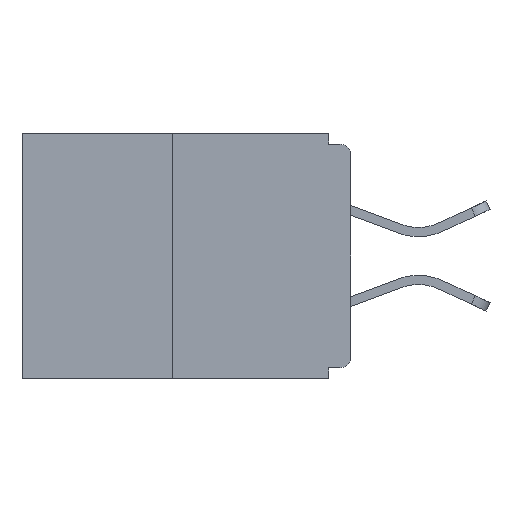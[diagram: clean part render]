
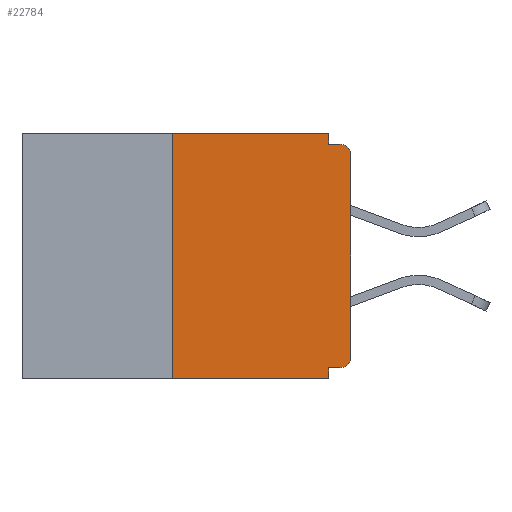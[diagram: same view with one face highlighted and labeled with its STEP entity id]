
A CAD part, left-side view. The second image highlights one B-rep face of the part: STEP entity #22784.
In plain terms, the highlighted planar face has unit normal (-1, 0, 0).
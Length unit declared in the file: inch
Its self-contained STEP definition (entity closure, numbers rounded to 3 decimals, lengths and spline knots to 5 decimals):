
#1736 = VECTOR ( 'NONE', #16011, 39.37008 ) ;
#2512 = EDGE_CURVE ( 'NONE', #23177, #23229, #24678, .T. ) ;
#2514 = CARTESIAN_POINT ( 'NONE',  ( 0., 0., -0.328 ) ) ;
#2651 = ORIENTED_EDGE ( 'NONE', *, *, #11335, .T. ) ;
#2685 = VERTEX_POINT ( 'NONE', #9331 ) ;
#2817 = VECTOR ( 'NONE', #18271, 39.37008 ) ;
#3033 = CARTESIAN_POINT ( 'NONE',  ( 0., 0.46, 0. ) ) ;
#3277 = CARTESIAN_POINT ( 'NONE',  ( 0., 0., -0.015 ) ) ;
#3321 = FACE_OUTER_BOUND ( 'NONE', #11960, .T. ) ;
#3941 = VECTOR ( 'NONE', #11304, 39.37008 ) ;
#3977 = ORIENTED_EDGE ( 'NONE', *, *, #21995, .T. ) ;
#4447 = CARTESIAN_POINT ( 'NONE',  ( 0., 0.25, 0. ) ) ;
#5215 = LINE ( 'NONE', #18017, #1736 ) ;
#5472 = DIRECTION ( 'NONE',  ( 0., 0., -1. ) ) ;
#5698 = CARTESIAN_POINT ( 'NONE',  ( 0., 0., -0.313 ) ) ;
#6737 = VECTOR ( 'NONE', #20362, 39.37008 ) ;
#7822 = CARTESIAN_POINT ( 'NONE',  ( 0., 0.031, -0.015 ) ) ;
#7859 = CIRCLE ( 'NONE', #24499, 0.015 ) ;
#7979 = DIRECTION ( 'NONE',  ( 0., 0., -1. ) ) ;
#8328 = LINE ( 'NONE', #17872, #12357 ) ;
#8707 = VERTEX_POINT ( 'NONE', #10016 ) ;
#8752 = VECTOR ( 'NONE', #18551, 39.37008 ) ;
#8835 = DIRECTION ( 'NONE',  ( 0., -1., 0. ) ) ;
#9174 = CARTESIAN_POINT ( 'NONE',  ( 0., 0., -0.03 ) ) ;
#9191 = EDGE_CURVE ( 'NONE', #17887, #13040, #24194, .T. ) ;
#9331 = CARTESIAN_POINT ( 'NONE',  ( 0., 0.031, 0. ) ) ;
#9357 = CARTESIAN_POINT ( 'NONE',  ( 0., 0.031, -0.343 ) ) ;
#9508 = VERTEX_POINT ( 'NONE', #5698 ) ;
#9536 = CARTESIAN_POINT ( 'NONE',  ( 0., 0.015, -0.03 ) ) ;
#10016 = CARTESIAN_POINT ( 'NONE',  ( 0., 0.015, -0.015 ) ) ;
#10813 = LINE ( 'NONE', #3277, #3941 ) ;
#11076 = DIRECTION ( 'NONE',  ( -1., 0., 0. ) ) ;
#11100 = PLANE ( 'NONE',  #22730 ) ;
#11304 = DIRECTION ( 'NONE',  ( 0., -1., 0. ) ) ;
#11315 = VECTOR ( 'NONE', #25258, 39.37008 ) ;
#11335 = EDGE_CURVE ( 'NONE', #22792, #8707, #7859, .T. ) ;
#11513 = CIRCLE ( 'NONE', #14159, 0.015 ) ;
#11531 = DIRECTION ( 'NONE',  ( -1., 0., 0. ) ) ;
#11960 = EDGE_LOOP ( 'NONE', ( #24630, #25038, #15161, #14620, #16665, #3977, #21230, #2651, #14775, #18588 ) ) ;
#12357 = VECTOR ( 'NONE', #7979, 39.37008 ) ;
#13040 = VERTEX_POINT ( 'NONE', #9357 ) ;
#13171 = DIRECTION ( 'NONE',  ( 0., 0., -1. ) ) ;
#13267 = VERTEX_POINT ( 'NONE', #16827 ) ;
#14062 = EDGE_CURVE ( 'NONE', #9508, #22792, #5215, .T. ) ;
#14159 = AXIS2_PLACEMENT_3D ( 'NONE', #25051, #11076, #13171 ) ;
#14198 = VECTOR ( 'NONE', #8835, 39.37008 ) ;
#14461 = EDGE_CURVE ( 'NONE', #2685, #15388, #8328, .T. ) ;
#14620 = ORIENTED_EDGE ( 'NONE', *, *, #19984, .F. ) ;
#14775 = ORIENTED_EDGE ( 'NONE', *, *, #23456, .F. ) ;
#14817 = LINE ( 'NONE', #3033, #14198 ) ;
#15161 = ORIENTED_EDGE ( 'NONE', *, *, #9191, .T. ) ;
#15310 = DIRECTION ( 'NONE',  ( 0., 0., -1. ) ) ;
#15388 = VERTEX_POINT ( 'NONE', #7822 ) ;
#16011 = DIRECTION ( 'NONE',  ( 0., 0., 1. ) ) ;
#16406 = LINE ( 'NONE', #19322, #11315 ) ;
#16562 = CARTESIAN_POINT ( 'NONE',  ( 0., 0.25, -0.343 ) ) ;
#16665 = ORIENTED_EDGE ( 'NONE', *, *, #2512, .F. ) ;
#16827 = CARTESIAN_POINT ( 'NONE',  ( 0., 0.25, 0. ) ) ;
#17872 = CARTESIAN_POINT ( 'NONE',  ( 0., 0.031, 0. ) ) ;
#17887 = VERTEX_POINT ( 'NONE', #16562 ) ;
#18017 = CARTESIAN_POINT ( 'NONE',  ( 0., 0., 0. ) ) ;
#18271 = DIRECTION ( 'NONE',  ( 0., 0., 1. ) ) ;
#18460 = CARTESIAN_POINT ( 'NONE',  ( 0., 0.015, -0.328 ) ) ;
#18551 = DIRECTION ( 'NONE',  ( 0., 1., 0. ) ) ;
#18588 = ORIENTED_EDGE ( 'NONE', *, *, #14461, .F. ) ;
#19322 = CARTESIAN_POINT ( 'NONE',  ( 0., 0.031, -0.343 ) ) ;
#19984 = EDGE_CURVE ( 'NONE', #23229, #13040, #16406, .T. ) ;
#20270 = CARTESIAN_POINT ( 'NONE',  ( 0., 0.031, -0.328 ) ) ;
#20362 = DIRECTION ( 'NONE',  ( 0., -1., 0. ) ) ;
#21230 = ORIENTED_EDGE ( 'NONE', *, *, #14062, .T. ) ;
#21463 = EDGE_CURVE ( 'NONE', #17887, #13267, #25331, .T. ) ;
#21995 = EDGE_CURVE ( 'NONE', #23177, #9508, #11513, .T. ) ;
#22730 = AXIS2_PLACEMENT_3D ( 'NONE', #23051, #25155, #15310 ) ;
#22784 = ADVANCED_FACE ( 'NONE', ( #3321 ), #11100, .F. ) ;
#22792 = VERTEX_POINT ( 'NONE', #9174 ) ;
#23051 = CARTESIAN_POINT ( 'NONE',  ( 0., 0.46, 0. ) ) ;
#23177 = VERTEX_POINT ( 'NONE', #18460 ) ;
#23229 = VERTEX_POINT ( 'NONE', #20270 ) ;
#23456 = EDGE_CURVE ( 'NONE', #15388, #8707, #10813, .T. ) ;
#24194 = LINE ( 'NONE', #24268, #6737 ) ;
#24268 = CARTESIAN_POINT ( 'NONE',  ( 0., 0.46, -0.343 ) ) ;
#24499 = AXIS2_PLACEMENT_3D ( 'NONE', #9536, #11531, #5472 ) ;
#24630 = ORIENTED_EDGE ( 'NONE', *, *, #25516, .F. ) ;
#24678 = LINE ( 'NONE', #2514, #8752 ) ;
#25038 = ORIENTED_EDGE ( 'NONE', *, *, #21463, .F. ) ;
#25051 = CARTESIAN_POINT ( 'NONE',  ( 0., 0.015, -0.313 ) ) ;
#25155 = DIRECTION ( 'NONE',  ( 1., 0., 0. ) ) ;
#25258 = DIRECTION ( 'NONE',  ( 0., 0., -1. ) ) ;
#25331 = LINE ( 'NONE', #4447, #2817 ) ;
#25516 = EDGE_CURVE ( 'NONE', #13267, #2685, #14817, .T. ) ;
